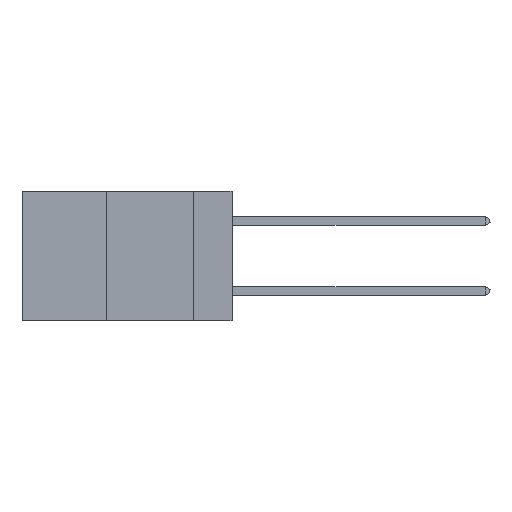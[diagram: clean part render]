
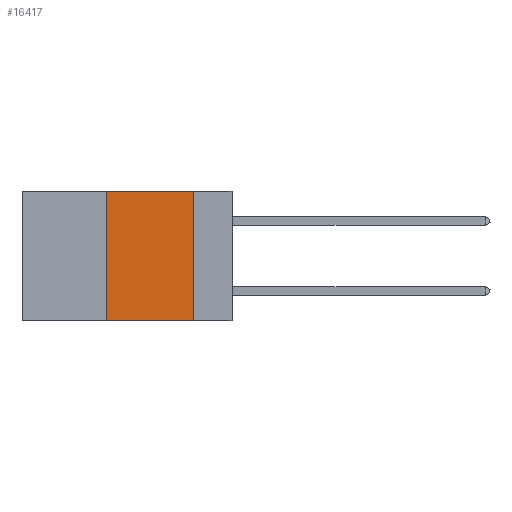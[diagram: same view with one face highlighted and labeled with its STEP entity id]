
A CAD part, left-side view. The second image highlights one B-rep face of the part: STEP entity #16417.
In plain terms, the highlighted planar face has unit normal (-1, 0, 0).
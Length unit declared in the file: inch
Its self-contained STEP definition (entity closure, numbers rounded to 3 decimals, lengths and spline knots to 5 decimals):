
#1617 = CARTESIAN_POINT ( 'NONE',  ( 0., 0.36, 0. ) ) ;
#1786 = VERTEX_POINT ( 'NONE', #1617 ) ;
#1895 = EDGE_CURVE ( 'NONE', #29398, #1786, #3376, .T. ) ;
#1947 = CARTESIAN_POINT ( 'NONE',  ( 0., 0.36, -0.37 ) ) ;
#2139 = DIRECTION ( 'NONE',  ( 0., 0., -1. ) ) ;
#3376 = LINE ( 'NONE', #4701, #35724 ) ;
#3394 = VERTEX_POINT ( 'NONE', #32833 ) ;
#3773 = VECTOR ( 'NONE', #8075, 39.37008 ) ;
#4701 = CARTESIAN_POINT ( 'NONE',  ( 0., 0.36, 0. ) ) ;
#7224 = ORIENTED_EDGE ( 'NONE', *, *, #30157, .F. ) ;
#7350 = CARTESIAN_POINT ( 'NONE',  ( 0., 0.11, -0.37 ) ) ;
#8075 = DIRECTION ( 'NONE',  ( 0., -1., 0. ) ) ;
#8949 = CARTESIAN_POINT ( 'NONE',  ( 0., 0.11, 0. ) ) ;
#12447 = LINE ( 'NONE', #8949, #28062 ) ;
#16417 = ADVANCED_FACE ( 'NONE', ( #19306 ), #17817, .F. ) ;
#17628 = ORIENTED_EDGE ( 'NONE', *, *, #1895, .F. ) ;
#17817 = PLANE ( 'NONE',  #29205 ) ;
#19306 = FACE_OUTER_BOUND ( 'NONE', #32931, .T. ) ;
#21069 = DIRECTION ( 'NONE',  ( 1., 0., 0. ) ) ;
#22293 = LINE ( 'NONE', #33857, #36860 ) ;
#24242 = DIRECTION ( 'NONE',  ( 0., 0., 1. ) ) ;
#25643 = VERTEX_POINT ( 'NONE', #7350 ) ;
#25881 = ORIENTED_EDGE ( 'NONE', *, *, #37138, .T. ) ;
#27159 = CARTESIAN_POINT ( 'NONE',  ( 0., 0.6, 0. ) ) ;
#28062 = VECTOR ( 'NONE', #40070, 39.37008 ) ;
#28843 = EDGE_CURVE ( 'NONE', #3394, #25643, #12447, .T. ) ;
#29205 = AXIS2_PLACEMENT_3D ( 'NONE', #27159, #21069, #2139 ) ;
#29398 = VERTEX_POINT ( 'NONE', #1947 ) ;
#29794 = LINE ( 'NONE', #33093, #3773 ) ;
#30157 = EDGE_CURVE ( 'NONE', #1786, #3394, #22293, .T. ) ;
#31205 = ORIENTED_EDGE ( 'NONE', *, *, #28843, .F. ) ;
#32833 = CARTESIAN_POINT ( 'NONE',  ( 0., 0.11, 0. ) ) ;
#32931 = EDGE_LOOP ( 'NONE', ( #31205, #7224, #17628, #25881 ) ) ;
#33093 = CARTESIAN_POINT ( 'NONE',  ( 0., 0.6, -0.37 ) ) ;
#33857 = CARTESIAN_POINT ( 'NONE',  ( 0., 0.6, 0. ) ) ;
#35724 = VECTOR ( 'NONE', #24242, 39.37008 ) ;
#36860 = VECTOR ( 'NONE', #36986, 39.37008 ) ;
#36986 = DIRECTION ( 'NONE',  ( 0., -1., 0. ) ) ;
#37138 = EDGE_CURVE ( 'NONE', #29398, #25643, #29794, .T. ) ;
#40070 = DIRECTION ( 'NONE',  ( 0., 0., -1. ) ) ;
